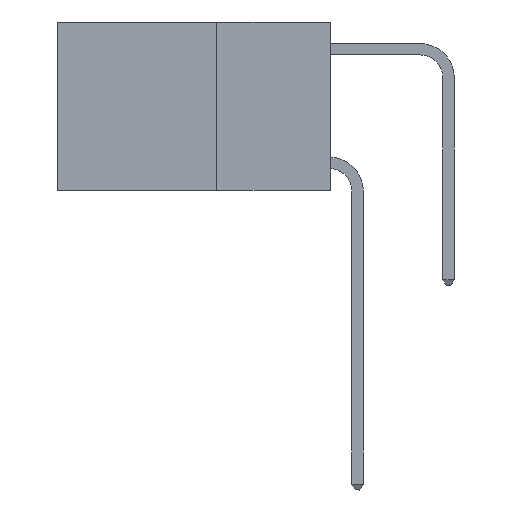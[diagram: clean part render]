
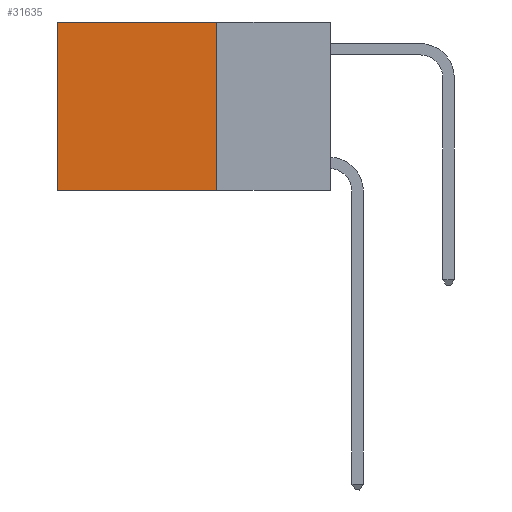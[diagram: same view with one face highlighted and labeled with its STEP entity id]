
A CAD part, left-side view. The second image highlights one B-rep face of the part: STEP entity #31635.
In plain terms, the highlighted planar face has unit normal (-1, 0, 0).
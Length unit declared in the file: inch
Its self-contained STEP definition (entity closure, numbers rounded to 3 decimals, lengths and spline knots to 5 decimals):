
#329 = VECTOR ( 'NONE', #33685, 39.37008 ) ;
#942 = LINE ( 'NONE', #21817, #24014 ) ;
#1697 = DIRECTION ( 'NONE',  ( 0., 1., 0. ) ) ;
#2173 = CARTESIAN_POINT ( 'NONE',  ( 0.2625, 0.25, -0.37 ) ) ;
#3603 = VERTEX_POINT ( 'NONE', #33356 ) ;
#4103 = CARTESIAN_POINT ( 'NONE',  ( 0.2625, 0.25, -0.37 ) ) ;
#4619 = DIRECTION ( 'NONE',  ( 0., 0., -1. ) ) ;
#5568 = ORIENTED_EDGE ( 'NONE', *, *, #18253, .F. ) ;
#6132 = EDGE_CURVE ( 'NONE', #10129, #3603, #6465, .T. ) ;
#6465 = LINE ( 'NONE', #4103, #31796 ) ;
#6852 = CARTESIAN_POINT ( 'NONE',  ( 0.2625, 0.25, 0. ) ) ;
#10129 = VERTEX_POINT ( 'NONE', #2173 ) ;
#11651 = DIRECTION ( 'NONE',  ( 0., 0., -1. ) ) ;
#12836 = EDGE_LOOP ( 'NONE', ( #30166, #27843, #5568, #20002 ) ) ;
#13258 = EDGE_CURVE ( 'NONE', #30390, #3603, #942, .T. ) ;
#17197 = VECTOR ( 'NONE', #22652, 39.37008 ) ;
#17454 = LINE ( 'NONE', #6852, #17197 ) ;
#18253 = EDGE_CURVE ( 'NONE', #28768, #10129, #17454, .T. ) ;
#18398 = CARTESIAN_POINT ( 'NONE',  ( 0.2625, 0.25, 0. ) ) ;
#19472 = LINE ( 'NONE', #18398, #329 ) ;
#20002 = ORIENTED_EDGE ( 'NONE', *, *, #29414, .T. ) ;
#20022 = PLANE ( 'NONE',  #27883 ) ;
#21817 = CARTESIAN_POINT ( 'NONE',  ( 0.2625, 0.6, 0. ) ) ;
#22652 = DIRECTION ( 'NONE',  ( 0., 0., -1. ) ) ;
#23280 = FACE_OUTER_BOUND ( 'NONE', #12836, .T. ) ;
#24014 = VECTOR ( 'NONE', #11651, 39.37008 ) ;
#24057 = CARTESIAN_POINT ( 'NONE',  ( 0.2625, 0.25, 0. ) ) ;
#25640 = CARTESIAN_POINT ( 'NONE',  ( 0.2625, 0.6, 0. ) ) ;
#27843 = ORIENTED_EDGE ( 'NONE', *, *, #6132, .F. ) ;
#27883 = AXIS2_PLACEMENT_3D ( 'NONE', #33725, #28102, #4619 ) ;
#28102 = DIRECTION ( 'NONE',  ( 1., 0., 0. ) ) ;
#28768 = VERTEX_POINT ( 'NONE', #24057 ) ;
#29414 = EDGE_CURVE ( 'NONE', #28768, #30390, #19472, .T. ) ;
#30166 = ORIENTED_EDGE ( 'NONE', *, *, #13258, .T. ) ;
#30390 = VERTEX_POINT ( 'NONE', #25640 ) ;
#31635 = ADVANCED_FACE ( 'NONE', ( #23280 ), #20022, .F. ) ;
#31796 = VECTOR ( 'NONE', #1697, 39.37008 ) ;
#33356 = CARTESIAN_POINT ( 'NONE',  ( 0.2625, 0.6, -0.37 ) ) ;
#33685 = DIRECTION ( 'NONE',  ( 0., 1., 0. ) ) ;
#33725 = CARTESIAN_POINT ( 'NONE',  ( 0.2625, 0.25, 0. ) ) ;
